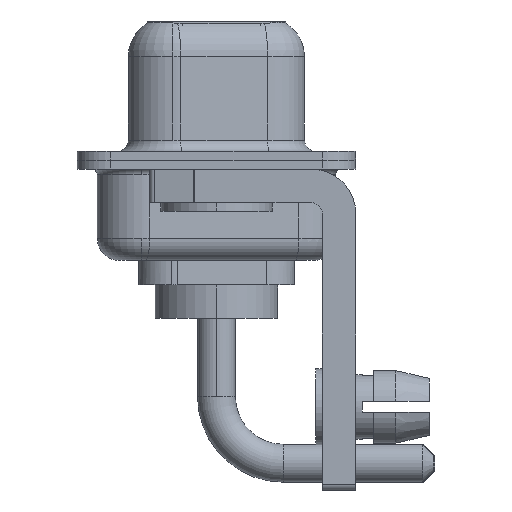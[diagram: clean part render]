
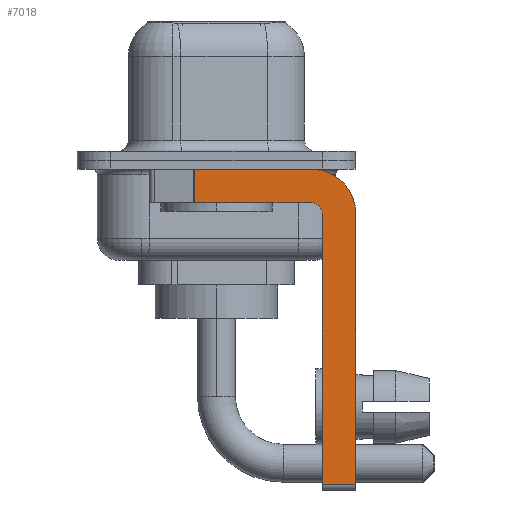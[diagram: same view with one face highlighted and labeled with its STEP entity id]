
A CAD part, left-side view. The second image highlights one B-rep face of the part: STEP entity #7018.
In plain terms, the highlighted planar face has unit normal (-1, 0, 0).
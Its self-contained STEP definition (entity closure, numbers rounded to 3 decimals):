
#185 = CARTESIAN_POINT ( 'NONE',  ( -2.9, -4.25, -14.55 ) ) ;
#261 = CARTESIAN_POINT ( 'NONE',  ( -2.9, -4.25, -1.9 ) ) ;
#357 = VECTOR ( 'NONE', #3583, 1000. ) ;
#500 = ORIENTED_EDGE ( 'NONE', *, *, #13043, .T. ) ;
#509 = DIRECTION ( 'NONE',  ( 0., 0., -1. ) ) ;
#512 = CIRCLE ( 'NONE', #4069, 0.5 ) ;
#741 = DIRECTION ( 'NONE',  ( 1., 0., 0. ) ) ;
#760 = LINE ( 'NONE', #15051, #13873 ) ;
#1242 = LINE ( 'NONE', #4977, #8706 ) ;
#1308 = DIRECTION ( 'NONE',  ( 0., 1., 0. ) ) ;
#1376 = LINE ( 'NONE', #185, #11657 ) ;
#1754 = DIRECTION ( 'NONE',  ( 1., 0., 0. ) ) ;
#1789 = VERTEX_POINT ( 'NONE', #2661 ) ;
#2387 = LINE ( 'NONE', #4769, #357 ) ;
#2395 = CARTESIAN_POINT ( 'NONE',  ( -2.9, -6.25, -2.4 ) ) ;
#2405 = DIRECTION ( 'NONE',  ( -1., 0., 0. ) ) ;
#2661 = CARTESIAN_POINT ( 'NONE',  ( -2.9, 0.978, -0.4 ) ) ;
#2831 = CIRCLE ( 'NONE', #11711, 2. ) ;
#2961 = FACE_OUTER_BOUND ( 'NONE', #9792, .T. ) ;
#2983 = DIRECTION ( 'NONE',  ( 0., 0., -1. ) ) ;
#3013 = ORIENTED_EDGE ( 'NONE', *, *, #7985, .F. ) ;
#3583 = DIRECTION ( 'NONE',  ( 0., 0., -1. ) ) ;
#3604 = CARTESIAN_POINT ( 'NONE',  ( -2.9, -6.25, -14.55 ) ) ;
#3642 = EDGE_CURVE ( 'NONE', #11866, #9607, #1242, .T. ) ;
#3723 = CARTESIAN_POINT ( 'NONE',  ( -2.9, 0.978, -1.9 ) ) ;
#3785 = ORIENTED_EDGE ( 'NONE', *, *, #3642, .F. ) ;
#4069 = AXIS2_PLACEMENT_3D ( 'NONE', #9390, #2405, #14234 ) ;
#4400 = VERTEX_POINT ( 'NONE', #3723 ) ;
#4769 = CARTESIAN_POINT ( 'NONE',  ( -2.9, -6.25, -2.4 ) ) ;
#4959 = DIRECTION ( 'NONE',  ( 0., -1., 0. ) ) ;
#4977 = CARTESIAN_POINT ( 'NONE',  ( -2.9, -4.75, -14.8 ) ) ;
#5597 = EDGE_CURVE ( 'NONE', #12164, #10214, #2387, .T. ) ;
#5783 = ORIENTED_EDGE ( 'NONE', *, *, #5597, .F. ) ;
#6004 = VECTOR ( 'NONE', #1308, 1000. ) ;
#6479 = AXIS2_PLACEMENT_3D ( 'NONE', #12643, #1754, #14307 ) ;
#7018 = ADVANCED_FACE ( 'NONE', ( #2961 ), #7805, .F. ) ;
#7276 = ORIENTED_EDGE ( 'NONE', *, *, #15123, .F. ) ;
#7343 = CARTESIAN_POINT ( 'NONE',  ( -2.9, 3., -0.4 ) ) ;
#7804 = ORIENTED_EDGE ( 'NONE', *, *, #8007, .F. ) ;
#7805 = PLANE ( 'NONE',  #6479 ) ;
#7985 = EDGE_CURVE ( 'NONE', #1789, #13714, #14408, .T. ) ;
#8007 = EDGE_CURVE ( 'NONE', #11623, #4400, #9639, .T. ) ;
#8706 = VECTOR ( 'NONE', #12037, 1000. ) ;
#9390 = CARTESIAN_POINT ( 'NONE',  ( -2.9, -4.25, -2.4 ) ) ;
#9607 = VERTEX_POINT ( 'NONE', #10932 ) ;
#9639 = LINE ( 'NONE', #12189, #6004 ) ;
#9792 = EDGE_LOOP ( 'NONE', ( #3013, #10370, #7804, #7276, #3785, #500, #5783, #10477 ) ) ;
#10214 = VERTEX_POINT ( 'NONE', #3604 ) ;
#10370 = ORIENTED_EDGE ( 'NONE', *, *, #10808, .T. ) ;
#10477 = ORIENTED_EDGE ( 'NONE', *, *, #14846, .F. ) ;
#10808 = EDGE_CURVE ( 'NONE', #1789, #4400, #760, .T. ) ;
#10932 = CARTESIAN_POINT ( 'NONE',  ( -2.9, -4.75, -2.4 ) ) ;
#11214 = CARTESIAN_POINT ( 'NONE',  ( -2.9, -4.75, -14.55 ) ) ;
#11510 = CARTESIAN_POINT ( 'NONE',  ( -2.9, -4.25, -0.4 ) ) ;
#11623 = VERTEX_POINT ( 'NONE', #261 ) ;
#11657 = VECTOR ( 'NONE', #4959, 1000. ) ;
#11711 = AXIS2_PLACEMENT_3D ( 'NONE', #14073, #741, #509 ) ;
#11866 = VERTEX_POINT ( 'NONE', #11214 ) ;
#12037 = DIRECTION ( 'NONE',  ( 0., 0., 1. ) ) ;
#12108 = DIRECTION ( 'NONE',  ( 0., -1., 0. ) ) ;
#12164 = VERTEX_POINT ( 'NONE', #2395 ) ;
#12189 = CARTESIAN_POINT ( 'NONE',  ( -2.9, -4.25, -1.9 ) ) ;
#12643 = CARTESIAN_POINT ( 'NONE',  ( -2.9, -4.25, -2.4 ) ) ;
#13043 = EDGE_CURVE ( 'NONE', #11866, #10214, #1376, .T. ) ;
#13714 = VERTEX_POINT ( 'NONE', #11510 ) ;
#13873 = VECTOR ( 'NONE', #2983, 1000. ) ;
#14073 = CARTESIAN_POINT ( 'NONE',  ( -2.9, -4.25, -2.4 ) ) ;
#14107 = VECTOR ( 'NONE', #12108, 1000. ) ;
#14234 = DIRECTION ( 'NONE',  ( 0., 0., 1. ) ) ;
#14307 = DIRECTION ( 'NONE',  ( 0., 0., -1. ) ) ;
#14408 = LINE ( 'NONE', #7343, #14107 ) ;
#14846 = EDGE_CURVE ( 'NONE', #13714, #12164, #2831, .T. ) ;
#15051 = CARTESIAN_POINT ( 'NONE',  ( -2.9, 0.978, -1.9 ) ) ;
#15123 = EDGE_CURVE ( 'NONE', #9607, #11623, #512, .T. ) ;
